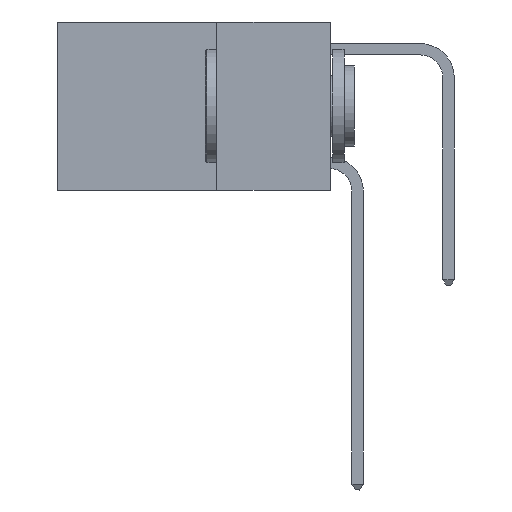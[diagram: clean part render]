
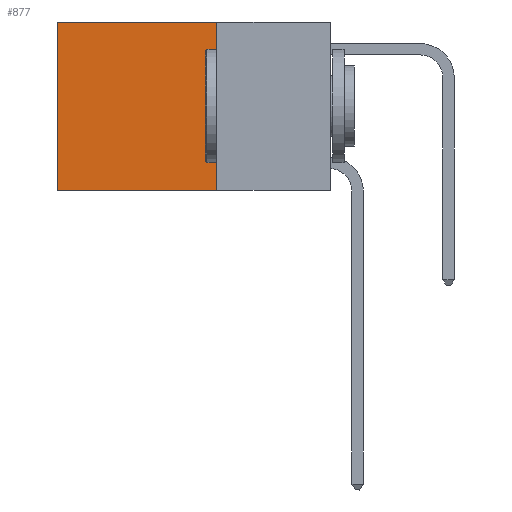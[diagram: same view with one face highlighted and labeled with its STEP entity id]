
A CAD part, left-side view. The second image highlights one B-rep face of the part: STEP entity #877.
In plain terms, the highlighted planar face has unit normal (-1, 0, 0).
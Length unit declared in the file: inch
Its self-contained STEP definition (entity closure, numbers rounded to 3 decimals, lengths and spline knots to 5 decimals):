
#440 = EDGE_CURVE ( 'NONE', #2551, #8499, #3068, .T. ) ;
#877 = ADVANCED_FACE ( 'NONE', ( #11171 ), #6390, .F. ) ;
#941 = LINE ( 'NONE', #12148, #16895 ) ;
#1457 = CARTESIAN_POINT ( 'NONE',  ( 0.2625, 0.6, 0. ) ) ;
#1655 = AXIS2_PLACEMENT_3D ( 'NONE', #8314, #21364, #10218 ) ;
#2551 = VERTEX_POINT ( 'NONE', #1457 ) ;
#2985 = EDGE_CURVE ( 'NONE', #22320, #2551, #5784, .T. ) ;
#3068 = LINE ( 'NONE', #12018, #18237 ) ;
#3336 = ORIENTED_EDGE ( 'NONE', *, *, #7520, .F. ) ;
#3346 = VECTOR ( 'NONE', #6328, 39.37008 ) ;
#4698 = DIRECTION ( 'NONE',  ( 0., 1., 0. ) ) ;
#5784 = LINE ( 'NONE', #21642, #15841 ) ;
#6328 = DIRECTION ( 'NONE',  ( 0., 1., 0. ) ) ;
#6390 = PLANE ( 'NONE',  #1655 ) ;
#7323 = LINE ( 'NONE', #15811, #3346 ) ;
#7520 = EDGE_CURVE ( 'NONE', #19429, #8499, #7323, .T. ) ;
#8314 = CARTESIAN_POINT ( 'NONE',  ( 0.2625, 0.25, 0. ) ) ;
#8499 = VERTEX_POINT ( 'NONE', #13400 ) ;
#9086 = ORIENTED_EDGE ( 'NONE', *, *, #10767, .F. ) ;
#10218 = DIRECTION ( 'NONE',  ( 0., 0., -1. ) ) ;
#10767 = EDGE_CURVE ( 'NONE', #22320, #19429, #941, .T. ) ;
#10908 = DIRECTION ( 'NONE',  ( 0., 0., -1. ) ) ;
#11171 = FACE_OUTER_BOUND ( 'NONE', #14070, .T. ) ;
#12018 = CARTESIAN_POINT ( 'NONE',  ( 0.2625, 0.6, 0. ) ) ;
#12148 = CARTESIAN_POINT ( 'NONE',  ( 0.2625, 0.25, 0. ) ) ;
#13400 = CARTESIAN_POINT ( 'NONE',  ( 0.2625, 0.6, -0.37 ) ) ;
#14070 = EDGE_LOOP ( 'NONE', ( #22784, #3336, #9086, #14100 ) ) ;
#14100 = ORIENTED_EDGE ( 'NONE', *, *, #2985, .T. ) ;
#15175 = CARTESIAN_POINT ( 'NONE',  ( 0.2625, 0.25, -0.37 ) ) ;
#15811 = CARTESIAN_POINT ( 'NONE',  ( 0.2625, 0.25, -0.37 ) ) ;
#15841 = VECTOR ( 'NONE', #4698, 39.37008 ) ;
#16895 = VECTOR ( 'NONE', #23274, 39.37008 ) ;
#18237 = VECTOR ( 'NONE', #10908, 39.37008 ) ;
#19038 = CARTESIAN_POINT ( 'NONE',  ( 0.2625, 0.25, 0. ) ) ;
#19429 = VERTEX_POINT ( 'NONE', #15175 ) ;
#21364 = DIRECTION ( 'NONE',  ( 1., 0., 0. ) ) ;
#21642 = CARTESIAN_POINT ( 'NONE',  ( 0.2625, 0.25, 0. ) ) ;
#22320 = VERTEX_POINT ( 'NONE', #19038 ) ;
#22784 = ORIENTED_EDGE ( 'NONE', *, *, #440, .T. ) ;
#23274 = DIRECTION ( 'NONE',  ( 0., 0., -1. ) ) ;
